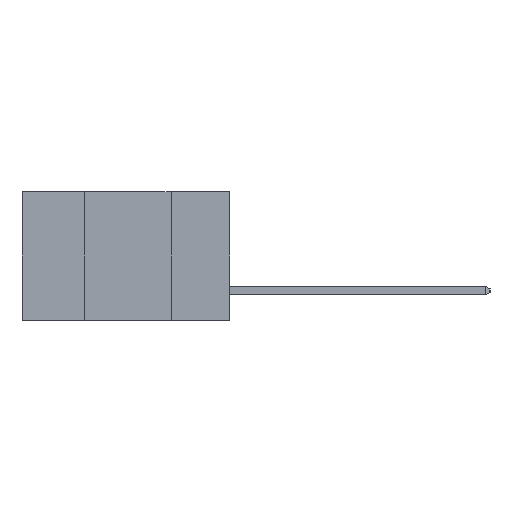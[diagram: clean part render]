
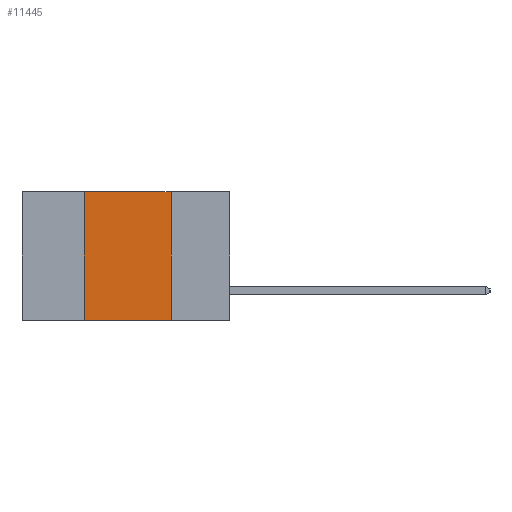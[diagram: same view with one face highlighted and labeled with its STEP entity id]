
A CAD part, left-side view. The second image highlights one B-rep face of the part: STEP entity #11445.
In plain terms, the highlighted planar face has unit normal (-1, 0, 0).
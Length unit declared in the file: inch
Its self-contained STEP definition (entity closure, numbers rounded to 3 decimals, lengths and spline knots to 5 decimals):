
#382 = CARTESIAN_POINT ( 'NONE',  ( 0., 0.42, 0. ) ) ;
#918 = CARTESIAN_POINT ( 'NONE',  ( 0., 0.6, 0. ) ) ;
#1452 = VERTEX_POINT ( 'NONE', #3729 ) ;
#1568 = CARTESIAN_POINT ( 'NONE',  ( 0., 0.17, 0. ) ) ;
#1667 = ORIENTED_EDGE ( 'NONE', *, *, #2181, .F. ) ;
#1800 = LINE ( 'NONE', #11407, #4400 ) ;
#1830 = ORIENTED_EDGE ( 'NONE', *, *, #11584, .T. ) ;
#2012 = DIRECTION ( 'NONE',  ( 1., 0., 0. ) ) ;
#2181 = EDGE_CURVE ( 'NONE', #11786, #1452, #1800, .T. ) ;
#2592 = ORIENTED_EDGE ( 'NONE', *, *, #9555, .F. ) ;
#2638 = VERTEX_POINT ( 'NONE', #9593 ) ;
#3047 = ORIENTED_EDGE ( 'NONE', *, *, #12262, .F. ) ;
#3370 = DIRECTION ( 'NONE',  ( 0., -1., 0. ) ) ;
#3398 = VECTOR ( 'NONE', #4308, 39.37008 ) ;
#3729 = CARTESIAN_POINT ( 'NONE',  ( 0., 0.17, -0.37 ) ) ;
#4266 = CARTESIAN_POINT ( 'NONE',  ( 0., 0.42, 0. ) ) ;
#4308 = DIRECTION ( 'NONE',  ( 0., -1., 0. ) ) ;
#4400 = VECTOR ( 'NONE', #4474, 39.37008 ) ;
#4474 = DIRECTION ( 'NONE',  ( 0., 0., -1. ) ) ;
#5495 = CARTESIAN_POINT ( 'NONE',  ( 0., 0.6, -0.37 ) ) ;
#5505 = VECTOR ( 'NONE', #9955, 39.37008 ) ;
#5880 = VERTEX_POINT ( 'NONE', #4266 ) ;
#6385 = FACE_OUTER_BOUND ( 'NONE', #10609, .T. ) ;
#6861 = LINE ( 'NONE', #5495, #11952 ) ;
#7383 = PLANE ( 'NONE',  #11149 ) ;
#8293 = LINE ( 'NONE', #382, #5505 ) ;
#9007 = LINE ( 'NONE', #11531, #3398 ) ;
#9445 = DIRECTION ( 'NONE',  ( 0., 0., -1. ) ) ;
#9555 = EDGE_CURVE ( 'NONE', #5880, #11786, #9007, .T. ) ;
#9593 = CARTESIAN_POINT ( 'NONE',  ( 0., 0.42, -0.37 ) ) ;
#9955 = DIRECTION ( 'NONE',  ( 0., 0., 1. ) ) ;
#10609 = EDGE_LOOP ( 'NONE', ( #1667, #2592, #3047, #1830 ) ) ;
#11149 = AXIS2_PLACEMENT_3D ( 'NONE', #918, #2012, #9445 ) ;
#11407 = CARTESIAN_POINT ( 'NONE',  ( 0., 0.17, 0. ) ) ;
#11445 = ADVANCED_FACE ( 'NONE', ( #6385 ), #7383, .F. ) ;
#11531 = CARTESIAN_POINT ( 'NONE',  ( 0., 0.6, 0. ) ) ;
#11584 = EDGE_CURVE ( 'NONE', #2638, #1452, #6861, .T. ) ;
#11786 = VERTEX_POINT ( 'NONE', #1568 ) ;
#11952 = VECTOR ( 'NONE', #3370, 39.37008 ) ;
#12262 = EDGE_CURVE ( 'NONE', #2638, #5880, #8293, .T. ) ;
